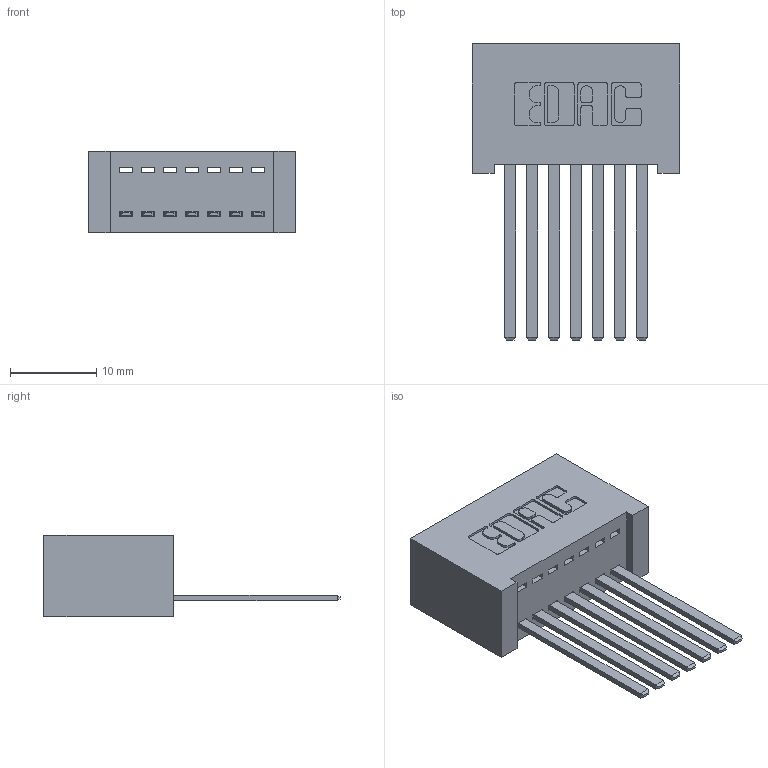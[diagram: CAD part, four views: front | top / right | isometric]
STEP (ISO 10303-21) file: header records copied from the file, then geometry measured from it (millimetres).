
FILE_DESCRIPTION (( 'STEP AP203' ), '1' );
FILE_NAME ('342-007-544-101.STEP', '2019-10-01T12:55:23', ( '' ), ( '' ), 'SwSTEP 2.0', 'SolidWorks 2016', '' );
FILE_SCHEMA (( 'CONFIG_CONTROL_DESIGN' ));
Length unit declared in the file: inch
Products named in the file (3): 342 Part_Lugless; 345-292-001_345-293-144; 342-007-544-101
Assembly tree (8 placements, depth 2):
  342-007-544-101
    342 Part_Lugless
    345-292-001_345-293-144  x7
Bounding box: 24.03 x 34.3 x 9.4 mm (x, y, z)
Volume: 2467.9 mm3; surface area: 3524.6 mm2
Topology: 8 solids, 8 shells, 466 faces, 1381 edges, 910 vertices
Faces by surface type: plane 328, cylinder 138
Entity records: 8213 total; most frequent: CARTESIAN_POINT 1427, ORIENTED_EDGE 1370, DIRECTION 1263, EDGE_CURVE 685, LINE 569, VECTOR 569, VERTEX_POINT 454, AXIS2_PLACEMENT_3D 347
